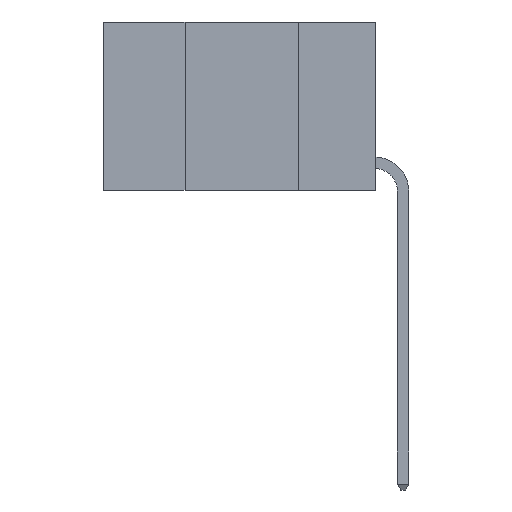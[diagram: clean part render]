
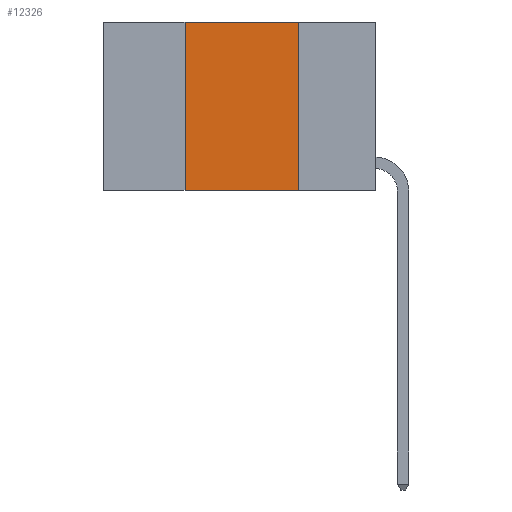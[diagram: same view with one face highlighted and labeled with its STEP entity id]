
A CAD part, left-side view. The second image highlights one B-rep face of the part: STEP entity #12326.
In plain terms, the highlighted planar face has unit normal (-1, 0, 0).
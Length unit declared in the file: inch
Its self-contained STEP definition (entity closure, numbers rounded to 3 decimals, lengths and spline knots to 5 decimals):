
#38 = CARTESIAN_POINT ( 'NONE',  ( 0., 0.6, -0.37 ) ) ;
#446 = ORIENTED_EDGE ( 'NONE', *, *, #6800, .F. ) ;
#1363 = DIRECTION ( 'NONE',  ( 0., -1., 0. ) ) ;
#1785 = VECTOR ( 'NONE', #10919, 39.37008 ) ;
#2515 = CARTESIAN_POINT ( 'NONE',  ( 0., 0.17, -0.37 ) ) ;
#3343 = DIRECTION ( 'NONE',  ( 1., 0., 0. ) ) ;
#3511 = CARTESIAN_POINT ( 'NONE',  ( 0., 0.17, 0. ) ) ;
#3521 = ORIENTED_EDGE ( 'NONE', *, *, #10729, .F. ) ;
#3913 = ORIENTED_EDGE ( 'NONE', *, *, #5054, .T. ) ;
#5054 = EDGE_CURVE ( 'NONE', #5625, #13219, #6232, .T. ) ;
#5625 = VERTEX_POINT ( 'NONE', #8956 ) ;
#5823 = VECTOR ( 'NONE', #1363, 39.37008 ) ;
#6169 = LINE ( 'NONE', #7600, #16092 ) ;
#6232 = LINE ( 'NONE', #38, #5823 ) ;
#6800 = EDGE_CURVE ( 'NONE', #5625, #10791, #6169, .T. ) ;
#7158 = PLANE ( 'NONE',  #16512 ) ;
#7600 = CARTESIAN_POINT ( 'NONE',  ( 0., 0.42, 0. ) ) ;
#8539 = EDGE_CURVE ( 'NONE', #16570, #13219, #16259, .T. ) ;
#8574 = EDGE_LOOP ( 'NONE', ( #13465, #3521, #446, #3913 ) ) ;
#8956 = CARTESIAN_POINT ( 'NONE',  ( 0., 0.42, -0.37 ) ) ;
#9625 = CARTESIAN_POINT ( 'NONE',  ( 0., 0.6, 0. ) ) ;
#10729 = EDGE_CURVE ( 'NONE', #10791, #16570, #15592, .T. ) ;
#10791 = VERTEX_POINT ( 'NONE', #11029 ) ;
#10919 = DIRECTION ( 'NONE',  ( 0., -1., 0. ) ) ;
#11029 = CARTESIAN_POINT ( 'NONE',  ( 0., 0.42, 0. ) ) ;
#11990 = CARTESIAN_POINT ( 'NONE',  ( 0., 0.17, 0. ) ) ;
#12326 = ADVANCED_FACE ( 'NONE', ( #15743 ), #7158, .F. ) ;
#12390 = DIRECTION ( 'NONE',  ( 0., 0., -1. ) ) ;
#12570 = DIRECTION ( 'NONE',  ( 0., 0., -1. ) ) ;
#12825 = DIRECTION ( 'NONE',  ( 0., 0., 1. ) ) ;
#13219 = VERTEX_POINT ( 'NONE', #2515 ) ;
#13234 = VECTOR ( 'NONE', #12570, 39.37008 ) ;
#13465 = ORIENTED_EDGE ( 'NONE', *, *, #8539, .F. ) ;
#14978 = CARTESIAN_POINT ( 'NONE',  ( 0., 0.6, 0. ) ) ;
#15592 = LINE ( 'NONE', #9625, #1785 ) ;
#15743 = FACE_OUTER_BOUND ( 'NONE', #8574, .T. ) ;
#16092 = VECTOR ( 'NONE', #12825, 39.37008 ) ;
#16259 = LINE ( 'NONE', #3511, #13234 ) ;
#16512 = AXIS2_PLACEMENT_3D ( 'NONE', #14978, #3343, #12390 ) ;
#16570 = VERTEX_POINT ( 'NONE', #11990 ) ;
